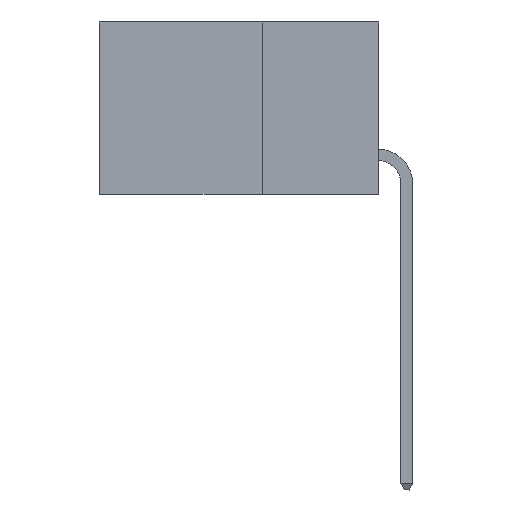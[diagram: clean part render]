
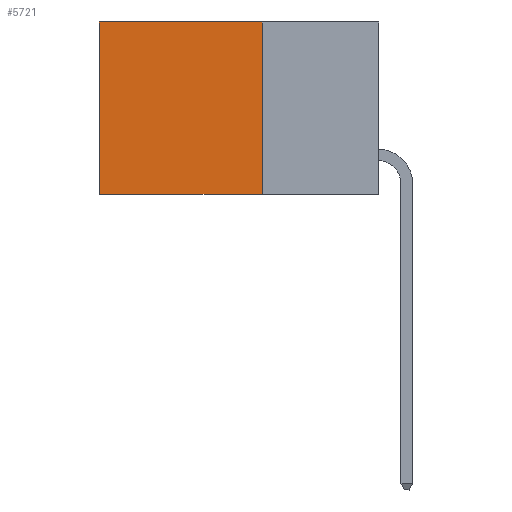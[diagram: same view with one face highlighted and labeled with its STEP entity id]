
A CAD part, left-side view. The second image highlights one B-rep face of the part: STEP entity #5721.
In plain terms, the highlighted planar face has unit normal (-1, 0, 0).
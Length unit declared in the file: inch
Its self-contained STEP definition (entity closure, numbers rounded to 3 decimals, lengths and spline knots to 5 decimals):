
#91 = EDGE_CURVE ( 'NONE', #1981, #1893, #10498, .T. ) ;
#365 = CARTESIAN_POINT ( 'NONE',  ( 0.298, 0.25, -0.37 ) ) ;
#526 = CARTESIAN_POINT ( 'NONE',  ( 0.298, 0.6, 0. ) ) ;
#1009 = VERTEX_POINT ( 'NONE', #365 ) ;
#1075 = DIRECTION ( 'NONE',  ( 1., 0., 0. ) ) ;
#1151 = DIRECTION ( 'NONE',  ( 0., 0., -1. ) ) ;
#1893 = VERTEX_POINT ( 'NONE', #6399 ) ;
#1973 = LINE ( 'NONE', #11457, #11119 ) ;
#1981 = VERTEX_POINT ( 'NONE', #526 ) ;
#2201 = CARTESIAN_POINT ( 'NONE',  ( 0.298, 0.25, 0. ) ) ;
#2338 = LINE ( 'NONE', #7447, #9114 ) ;
#2504 = ORIENTED_EDGE ( 'NONE', *, *, #3942, .T. ) ;
#2959 = VERTEX_POINT ( 'NONE', #11459 ) ;
#3832 = LINE ( 'NONE', #4612, #10576 ) ;
#3942 = EDGE_CURVE ( 'NONE', #2959, #1981, #1973, .T. ) ;
#4612 = CARTESIAN_POINT ( 'NONE',  ( 0.298, 0.25, 0. ) ) ;
#4771 = ORIENTED_EDGE ( 'NONE', *, *, #6769, .F. ) ;
#5229 = PLANE ( 'NONE',  #10482 ) ;
#5362 = DIRECTION ( 'NONE',  ( 0., 1., 0. ) ) ;
#5721 = ADVANCED_FACE ( 'NONE', ( #8226 ), #5229, .F. ) ;
#6330 = EDGE_LOOP ( 'NONE', ( #7299, #4771, #11326, #2504 ) ) ;
#6399 = CARTESIAN_POINT ( 'NONE',  ( 0.298, 0.6, -0.37 ) ) ;
#6734 = DIRECTION ( 'NONE',  ( 0., 0., -1. ) ) ;
#6760 = CARTESIAN_POINT ( 'NONE',  ( 0.298, 0.6, 0. ) ) ;
#6769 = EDGE_CURVE ( 'NONE', #1009, #1893, #2338, .T. ) ;
#7299 = ORIENTED_EDGE ( 'NONE', *, *, #91, .T. ) ;
#7447 = CARTESIAN_POINT ( 'NONE',  ( 0.298, 0.25, -0.37 ) ) ;
#8226 = FACE_OUTER_BOUND ( 'NONE', #6330, .T. ) ;
#8312 = DIRECTION ( 'NONE',  ( 0., 1., 0. ) ) ;
#8957 = DIRECTION ( 'NONE',  ( 0., 0., -1. ) ) ;
#9114 = VECTOR ( 'NONE', #8312, 39.37008 ) ;
#10118 = EDGE_CURVE ( 'NONE', #2959, #1009, #3832, .T. ) ;
#10201 = VECTOR ( 'NONE', #6734, 39.37008 ) ;
#10482 = AXIS2_PLACEMENT_3D ( 'NONE', #2201, #1075, #1151 ) ;
#10498 = LINE ( 'NONE', #6760, #10201 ) ;
#10576 = VECTOR ( 'NONE', #8957, 39.37008 ) ;
#11119 = VECTOR ( 'NONE', #5362, 39.37008 ) ;
#11326 = ORIENTED_EDGE ( 'NONE', *, *, #10118, .F. ) ;
#11457 = CARTESIAN_POINT ( 'NONE',  ( 0.298, 0.25, 0. ) ) ;
#11459 = CARTESIAN_POINT ( 'NONE',  ( 0.298, 0.25, 0. ) ) ;
